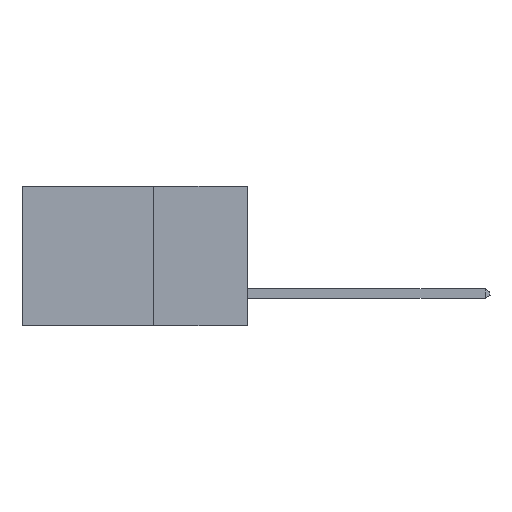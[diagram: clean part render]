
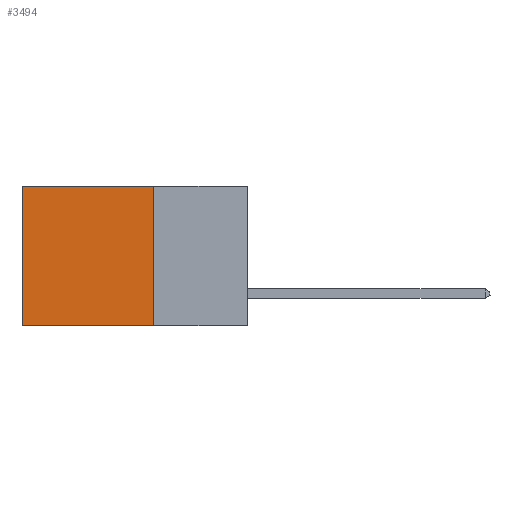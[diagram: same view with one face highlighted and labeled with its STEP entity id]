
A CAD part, left-side view. The second image highlights one B-rep face of the part: STEP entity #3494.
In plain terms, the highlighted planar face has unit normal (-1, 0, 0).
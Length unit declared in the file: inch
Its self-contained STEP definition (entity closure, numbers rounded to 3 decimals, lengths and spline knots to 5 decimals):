
#948 = CARTESIAN_POINT ( 'NONE',  ( 0.298, 0.6, 0. ) ) ;
#1609 = PLANE ( 'NONE',  #5911 ) ;
#1849 = DIRECTION ( 'NONE',  ( 0., 0., -1. ) ) ;
#1940 = CARTESIAN_POINT ( 'NONE',  ( 0.298, 0.25, 0. ) ) ;
#2766 = CARTESIAN_POINT ( 'NONE',  ( 0.298, 0.25, 0. ) ) ;
#2858 = VECTOR ( 'NONE', #1849, 39.37008 ) ;
#3346 = VECTOR ( 'NONE', #6006, 39.37008 ) ;
#3494 = ADVANCED_FACE ( 'NONE', ( #13142 ), #1609, .F. ) ;
#4098 = DIRECTION ( 'NONE',  ( 0., 1., 0. ) ) ;
#4108 = VECTOR ( 'NONE', #9287, 39.37008 ) ;
#4249 = VERTEX_POINT ( 'NONE', #2766 ) ;
#4335 = CARTESIAN_POINT ( 'NONE',  ( 0.298, 0.6, 0. ) ) ;
#4792 = CARTESIAN_POINT ( 'NONE',  ( 0.298, 0.25, 0. ) ) ;
#5911 = AXIS2_PLACEMENT_3D ( 'NONE', #4792, #6776, #8856 ) ;
#6006 = DIRECTION ( 'NONE',  ( 0., 1., 0. ) ) ;
#6015 = CARTESIAN_POINT ( 'NONE',  ( 0.298, 0.25, 0. ) ) ;
#6291 = VERTEX_POINT ( 'NONE', #4335 ) ;
#6730 = LINE ( 'NONE', #1940, #2858 ) ;
#6776 = DIRECTION ( 'NONE',  ( 1., 0., 0. ) ) ;
#6892 = CARTESIAN_POINT ( 'NONE',  ( 0.298, 0.25, -0.37 ) ) ;
#7289 = CARTESIAN_POINT ( 'NONE',  ( 0.298, 0.25, -0.37 ) ) ;
#7508 = EDGE_LOOP ( 'NONE', ( #11064, #9927, #7979, #11993 ) ) ;
#7979 = ORIENTED_EDGE ( 'NONE', *, *, #12454, .F. ) ;
#8151 = VECTOR ( 'NONE', #4098, 39.37008 ) ;
#8856 = DIRECTION ( 'NONE',  ( 0., 0., -1. ) ) ;
#9287 = DIRECTION ( 'NONE',  ( 0., 0., -1. ) ) ;
#9760 = CARTESIAN_POINT ( 'NONE',  ( 0.298, 0.6, -0.37 ) ) ;
#9927 = ORIENTED_EDGE ( 'NONE', *, *, #11742, .F. ) ;
#10576 = EDGE_CURVE ( 'NONE', #4249, #6291, #11913, .T. ) ;
#10604 = EDGE_CURVE ( 'NONE', #6291, #12926, #12384, .T. ) ;
#11064 = ORIENTED_EDGE ( 'NONE', *, *, #10604, .T. ) ;
#11742 = EDGE_CURVE ( 'NONE', #12665, #12926, #11779, .T. ) ;
#11779 = LINE ( 'NONE', #6892, #3346 ) ;
#11913 = LINE ( 'NONE', #6015, #8151 ) ;
#11993 = ORIENTED_EDGE ( 'NONE', *, *, #10576, .T. ) ;
#12384 = LINE ( 'NONE', #948, #4108 ) ;
#12454 = EDGE_CURVE ( 'NONE', #4249, #12665, #6730, .T. ) ;
#12665 = VERTEX_POINT ( 'NONE', #7289 ) ;
#12926 = VERTEX_POINT ( 'NONE', #9760 ) ;
#13142 = FACE_OUTER_BOUND ( 'NONE', #7508, .T. ) ;
